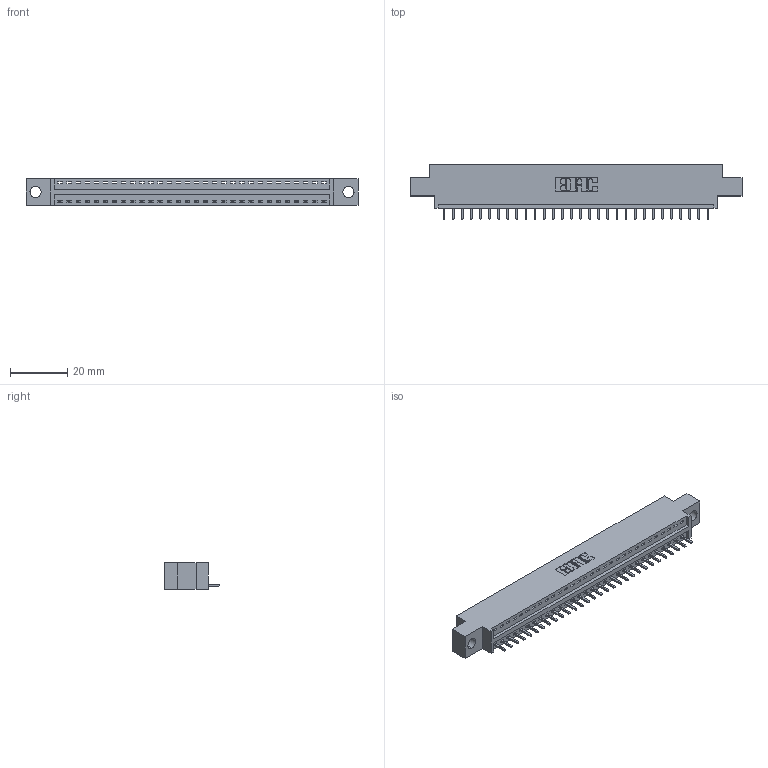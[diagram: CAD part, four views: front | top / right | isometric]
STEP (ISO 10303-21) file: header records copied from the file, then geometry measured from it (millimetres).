
FILE_DESCRIPTION (( 'STEP AP203' ), '1' );
FILE_NAME ('346-030-521-604.STEP', '2022-05-06T15:28:19', ( '' ), ( '' ), 'SwSTEP 2.0', 'SolidWorks 2020', '' );
FILE_SCHEMA (( 'CONFIG_CONTROL_DESIGN' ));
Length unit declared in the file: inch
Products named in the file (3): 345-292-001_345-293-121; 346 Part_0.170 Offset - 0.156 Dia-TH; 346-030-521-604
Assembly tree (31 placements, depth 2):
  346-030-521-604
    346 Part_0.170 Offset - 0.156 Dia-TH
    345-292-001_345-293-121  x30
Bounding box: 115.82 x 19.05 x 9.4 mm (x, y, z)
Volume: 10658.3 mm3; surface area: 12850.1 mm2
Topology: 31 solids, 31 shells, 1880 faces, 5657 edges, 3730 vertices
Faces by surface type: plane 1294, cylinder 586
Entity records: 20803 total; most frequent: CARTESIAN_POINT 3580, ORIENTED_EDGE 3542, DIRECTION 3171, EDGE_CURVE 1771, VECTOR 1519, LINE 1519, VERTEX_POINT 1178, AXIS2_PLACEMENT_3D 826
